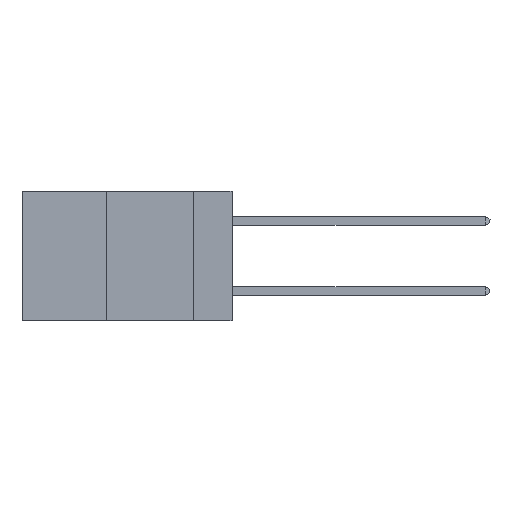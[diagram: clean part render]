
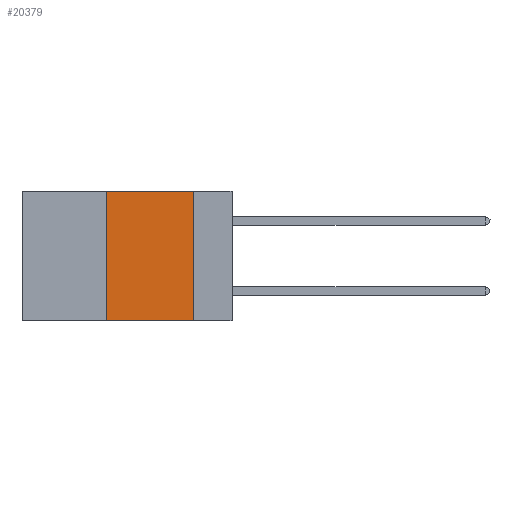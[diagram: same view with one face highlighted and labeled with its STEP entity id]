
A CAD part, left-side view. The second image highlights one B-rep face of the part: STEP entity #20379.
In plain terms, the highlighted planar face has unit normal (-1, 0, 0).
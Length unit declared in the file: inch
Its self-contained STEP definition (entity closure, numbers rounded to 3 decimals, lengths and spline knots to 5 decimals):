
#167 = DIRECTION ( 'NONE',  ( 0., 0., 1. ) ) ;
#713 = ORIENTED_EDGE ( 'NONE', *, *, #2752, .F. ) ;
#1605 = PLANE ( 'NONE',  #16628 ) ;
#1734 = LINE ( 'NONE', #18083, #9919 ) ;
#1760 = DIRECTION ( 'NONE',  ( 0., 0., -1. ) ) ;
#2670 = EDGE_CURVE ( 'NONE', #19633, #3993, #1734, .T. ) ;
#2752 = EDGE_CURVE ( 'NONE', #10063, #3993, #4488, .T. ) ;
#2845 = DIRECTION ( 'NONE',  ( 0., -1., 0. ) ) ;
#3638 = EDGE_CURVE ( 'NONE', #16901, #10063, #22385, .T. ) ;
#3993 = VERTEX_POINT ( 'NONE', #5422 ) ;
#4488 = LINE ( 'NONE', #4525, #17829 ) ;
#4525 = CARTESIAN_POINT ( 'NONE',  ( 0., 0.11, 0. ) ) ;
#5325 = CARTESIAN_POINT ( 'NONE',  ( 0., 0.11, 0. ) ) ;
#5422 = CARTESIAN_POINT ( 'NONE',  ( 0., 0.11, -0.37 ) ) ;
#7651 = DIRECTION ( 'NONE',  ( 0., -1., 0. ) ) ;
#8776 = ORIENTED_EDGE ( 'NONE', *, *, #3638, .F. ) ;
#9655 = CARTESIAN_POINT ( 'NONE',  ( 0., 0.6, 0. ) ) ;
#9866 = VECTOR ( 'NONE', #2845, 39.37008 ) ;
#9919 = VECTOR ( 'NONE', #7651, 39.37008 ) ;
#10063 = VERTEX_POINT ( 'NONE', #5325 ) ;
#10284 = ORIENTED_EDGE ( 'NONE', *, *, #2670, .T. ) ;
#10523 = CARTESIAN_POINT ( 'NONE',  ( 0., 0.36, 0. ) ) ;
#12190 = CARTESIAN_POINT ( 'NONE',  ( 0., 0.6, 0. ) ) ;
#12294 = CARTESIAN_POINT ( 'NONE',  ( 0., 0.36, -0.37 ) ) ;
#13288 = DIRECTION ( 'NONE',  ( 0., 0., -1. ) ) ;
#13533 = VECTOR ( 'NONE', #167, 39.37008 ) ;
#15344 = ORIENTED_EDGE ( 'NONE', *, *, #17252, .F. ) ;
#15851 = DIRECTION ( 'NONE',  ( 1., 0., 0. ) ) ;
#16628 = AXIS2_PLACEMENT_3D ( 'NONE', #12190, #15851, #1760 ) ;
#16901 = VERTEX_POINT ( 'NONE', #18046 ) ;
#17252 = EDGE_CURVE ( 'NONE', #19633, #16901, #22467, .T. ) ;
#17829 = VECTOR ( 'NONE', #13288, 39.37008 ) ;
#18046 = CARTESIAN_POINT ( 'NONE',  ( 0., 0.36, 0. ) ) ;
#18083 = CARTESIAN_POINT ( 'NONE',  ( 0., 0.6, -0.37 ) ) ;
#19633 = VERTEX_POINT ( 'NONE', #12294 ) ;
#19767 = FACE_OUTER_BOUND ( 'NONE', #21656, .T. ) ;
#20379 = ADVANCED_FACE ( 'NONE', ( #19767 ), #1605, .F. ) ;
#21656 = EDGE_LOOP ( 'NONE', ( #713, #8776, #15344, #10284 ) ) ;
#22385 = LINE ( 'NONE', #9655, #9866 ) ;
#22467 = LINE ( 'NONE', #10523, #13533 ) ;
